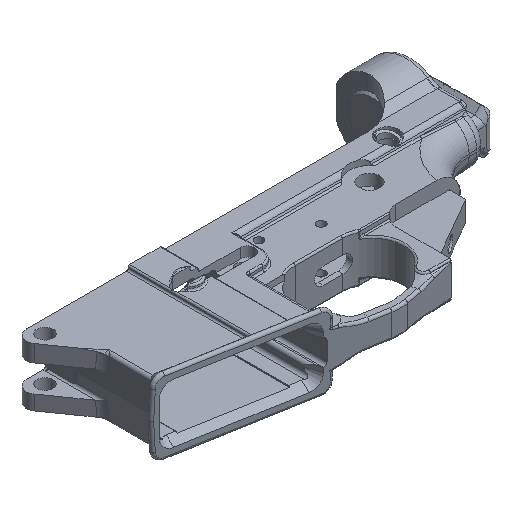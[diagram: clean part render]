
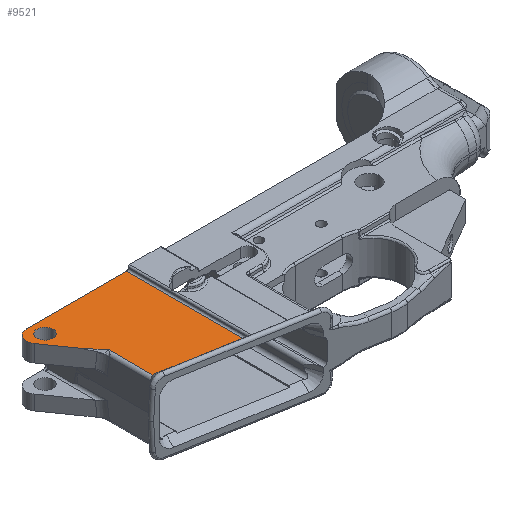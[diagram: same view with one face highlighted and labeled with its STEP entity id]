
A CAD part, isometric view. The second image highlights one B-rep face of the part: STEP entity #9521.
In plain terms, the highlighted planar face has unit normal (0, 0, 1).
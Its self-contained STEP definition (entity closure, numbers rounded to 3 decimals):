
#129=FACE_BOUND('',#1964,.T.);
#305=B_SPLINE_CURVE_WITH_KNOTS('',3,(#16987,#16988,#16989,#16990,#16991,
#16992),.UNSPECIFIED.,.F.,.F.,(4,2,4),(-0.114,-0.051,
0.),.UNSPECIFIED.);
#401=B_SPLINE_CURVE_WITH_KNOTS('',3,(#21925,#21926,#21927,#21928,#21929,
#21930,#21931,#21932,#21933,#21934,#21935,#21936,#21937,#21938),
 .UNSPECIFIED.,.F.,.F.,(4,2,2,2,2,2,4),(-0.993,-0.797,
-0.381,-0.24,-0.093,0.,0.017),
 .UNSPECIFIED.);
#879=PLANE('',#10477);
#1397=FACE_OUTER_BOUND('',#1963,.T.);
#1963=EDGE_LOOP('',(#8847,#8848,#8849,#8850,#8851,#8852,#8853,#8854));
#1964=EDGE_LOOP('',(#8855));
#2267=LINE('',#15436,#2973);
#2377=LINE('',#16474,#3083);
#2538=LINE('',#18590,#3244);
#2668=LINE('',#21567,#3374);
#2685=LINE('',#22036,#3391);
#2973=VECTOR('',#11481,35.853);
#3083=VECTOR('',#11819,54.9);
#3244=VECTOR('',#12424,20.718);
#3374=VECTOR('',#12996,10.);
#3391=VECTOR('',#13061,37.251);
#3702=CIRCLE('',#10236,3.738);
#3803=CIRCLE('',#10478,5.);
#4184=VERTEX_POINT('',#15433);
#4185=VERTEX_POINT('',#15435);
#4329=VERTEX_POINT('',#16472);
#4425=VERTEX_POINT('',#16986);
#4521=VERTEX_POINT('',#18456);
#4526=VERTEX_POINT('',#18594);
#4697=VERTEX_POINT('',#21557);
#4698=VERTEX_POINT('',#21560);
#4711=VERTEX_POINT('',#22034);
#5250=EDGE_CURVE('',#4184,#4185,#2267,.T.);
#5453=EDGE_CURVE('',#4329,#4184,#2377,.T.);
#5608=EDGE_CURVE('',#4185,#4425,#305,.T.);
#5780=EDGE_CURVE('',#4425,#4521,#2538,.T.);
#5783=EDGE_CURVE('',#4526,#4526,#3702,.T.);
#6094=EDGE_CURVE('',#4698,#4697,#2668,.T.);
#6095=EDGE_CURVE('',#4698,#4521,#401,.T.);
#6124=EDGE_CURVE('',#4697,#4711,#3803,.T.);
#6125=EDGE_CURVE('',#4711,#4329,#2685,.T.);
#8847=ORIENTED_EDGE('',*,*,#6124,.F.);
#8848=ORIENTED_EDGE('',*,*,#6094,.F.);
#8849=ORIENTED_EDGE('',*,*,#6095,.T.);
#8850=ORIENTED_EDGE('',*,*,#5780,.F.);
#8851=ORIENTED_EDGE('',*,*,#5608,.F.);
#8852=ORIENTED_EDGE('',*,*,#5250,.F.);
#8853=ORIENTED_EDGE('',*,*,#5453,.F.);
#8854=ORIENTED_EDGE('',*,*,#6125,.F.);
#8855=ORIENTED_EDGE('',*,*,#5783,.T.);
#9521=ADVANCED_FACE('',(#1397,#129),#879,.F.);
#10236=AXIS2_PLACEMENT_3D('',#18596,#12430,#12431);
#10477=AXIS2_PLACEMENT_3D('',#22033,#13057,#13058);
#10478=AXIS2_PLACEMENT_3D('',#22035,#13059,#13060);
#11481=DIRECTION('',(-0.985,0.174,0.));
#11819=DIRECTION('',(0.,-1.,0.));
#12424=DIRECTION('',(0.,1.,0.));
#12430=DIRECTION('center_axis',(0.,0.,
-1.));
#12431=DIRECTION('ref_axis',(0.,-1.,0.));
#12996=DIRECTION('',(-0.574,0.819,0.));
#13057=DIRECTION('center_axis',(0.,0.,
-1.));
#13058=DIRECTION('ref_axis',(0.,-1.,0.));
#13059=DIRECTION('center_axis',(0.,0.,
-1.));
#13060=DIRECTION('ref_axis',(0.,1.,0.));
#13061=DIRECTION('',(1.,0.,0.));
#15433=CARTESIAN_POINT('',(444.425,113.133,28.017));
#15435=CARTESIAN_POINT('',(409.116,119.359,28.017));
#15436=CARTESIAN_POINT('',(444.425,113.133,28.017));
#16472=CARTESIAN_POINT('',(444.425,168.033,28.017));
#16474=CARTESIAN_POINT('',(444.425,168.033,28.017));
#16986=CARTESIAN_POINT('',(408.113,119.207,28.017));
#16987=CARTESIAN_POINT('Ctrl Pts',(409.116,119.359,28.017));
#16988=CARTESIAN_POINT('Ctrl Pts',(408.978,119.383,28.017));
#16989=CARTESIAN_POINT('Ctrl Pts',(408.811,119.39,28.017));
#16990=CARTESIAN_POINT('Ctrl Pts',(408.437,119.324,28.017));
#16991=CARTESIAN_POINT('Ctrl Pts',(408.271,119.271,28.017));
#16992=CARTESIAN_POINT('Ctrl Pts',(408.113,119.207,28.017));
#18456=CARTESIAN_POINT('',(408.113,139.925,28.017));
#18590=CARTESIAN_POINT('',(408.113,119.207,28.017));
#18594=CARTESIAN_POINT('',(399.594,165.421,28.017));
#18596=CARTESIAN_POINT('Origin',(399.594,161.683,28.017));
#21557=CARTESIAN_POINT('',(393.011,160.165,28.017));
#21560=CARTESIAN_POINT('',(402.245,146.977,28.017));
#21567=CARTESIAN_POINT('',(412.142,132.844,28.017));
#21925=CARTESIAN_POINT('Ctrl Pts',(402.245,146.977,28.017));
#21926=CARTESIAN_POINT('Ctrl Pts',(402.546,146.596,28.017));
#21927=CARTESIAN_POINT('Ctrl Pts',(402.834,146.235,28.017));
#21928=CARTESIAN_POINT('Ctrl Pts',(403.955,144.841,28.017));
#21929=CARTESIAN_POINT('Ctrl Pts',(404.497,144.185,28.017));
#21930=CARTESIAN_POINT('Ctrl Pts',(405.715,142.754,28.017));
#21931=CARTESIAN_POINT('Ctrl Pts',(406.035,142.38,28.017));
#21932=CARTESIAN_POINT('Ctrl Pts',(406.741,141.551,28.017));
#21933=CARTESIAN_POINT('Ctrl Pts',(407.044,141.193,28.017));
#21934=CARTESIAN_POINT('Ctrl Pts',(407.591,140.545,28.017));
#21935=CARTESIAN_POINT('Ctrl Pts',(407.804,140.293,28.017));
#21936=CARTESIAN_POINT('Ctrl Pts',(408.041,140.012,28.017));
#21937=CARTESIAN_POINT('Ctrl Pts',(408.077,139.969,28.017));
#21938=CARTESIAN_POINT('Ctrl Pts',(408.113,139.925,28.017));
#22033=CARTESIAN_POINT('Origin',(419.723,112.804,28.017));
#22034=CARTESIAN_POINT('',(397.107,168.033,28.017));
#22035=CARTESIAN_POINT('Origin',(397.107,163.033,28.017));
#22036=CARTESIAN_POINT('',(407.173,168.033,28.017));
